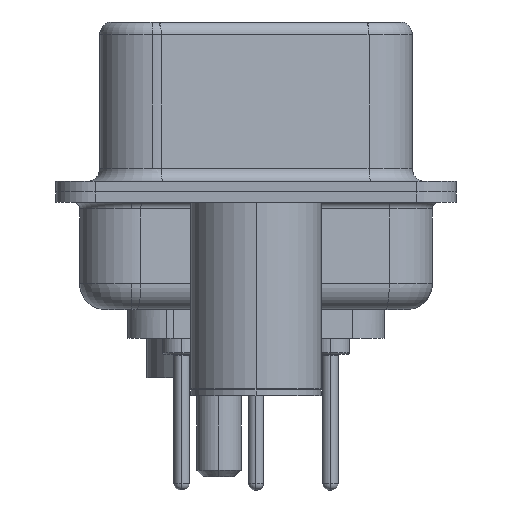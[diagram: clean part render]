
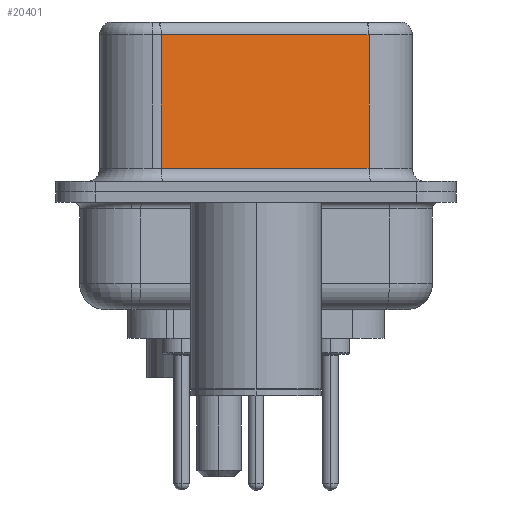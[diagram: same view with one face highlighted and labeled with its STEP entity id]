
A CAD part, left-side view. The second image highlights one B-rep face of the part: STEP entity #20401.
In plain terms, the highlighted planar face has unit normal (-0.985, -0.174, 0).
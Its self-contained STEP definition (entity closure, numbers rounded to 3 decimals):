
#1045 = AXIS2_PLACEMENT_3D ( 'NONE', #29341, #17605, #1717 ) ;
#1717 = DIRECTION ( 'NONE',  ( -0.174, 0.985, 0. ) ) ;
#2095 = CARTESIAN_POINT ( 'NONE',  ( 5.132, -4.322, 0.9 ) ) ;
#3301 = LINE ( 'NONE', #2095, #13790 ) ;
#3924 = CARTESIAN_POINT ( 'NONE',  ( 5.132, -4.322, 0.9 ) ) ;
#5317 = VERTEX_POINT ( 'NONE', #3924 ) ;
#5989 = EDGE_CURVE ( 'NONE', #20471, #5317, #24504, .T. ) ;
#6259 = PLANE ( 'NONE',  #1045 ) ;
#8406 = EDGE_CURVE ( 'NONE', #20471, #17214, #12701, .T. ) ;
#8495 = VECTOR ( 'NONE', #23700, 1000. ) ;
#9767 = DIRECTION ( 'NONE',  ( -0.174, 0.985, 0. ) ) ;
#10896 = CARTESIAN_POINT ( 'NONE',  ( 3.73, 3.628, 0.9 ) ) ;
#10901 = DIRECTION ( 'NONE',  ( 0.174, -0.985, 0. ) ) ;
#11089 = VECTOR ( 'NONE', #12993, 1000. ) ;
#11723 = CARTESIAN_POINT ( 'NONE',  ( 5.132, -4.322, 6.52 ) ) ;
#12054 = EDGE_CURVE ( 'NONE', #17214, #20458, #22404, .T. ) ;
#12107 = CARTESIAN_POINT ( 'NONE',  ( 5.132, -4.322, 6.02 ) ) ;
#12701 = LINE ( 'NONE', #12107, #25792 ) ;
#12714 = ORIENTED_EDGE ( 'NONE', *, *, #22358, .T. ) ;
#12993 = DIRECTION ( 'NONE',  ( 0., 0., -1. ) ) ;
#13790 = VECTOR ( 'NONE', #10901, 1000. ) ;
#15460 = CARTESIAN_POINT ( 'NONE',  ( 5.132, -4.322, 6.02 ) ) ;
#15573 = ORIENTED_EDGE ( 'NONE', *, *, #12054, .T. ) ;
#17214 = VERTEX_POINT ( 'NONE', #24211 ) ;
#17605 = DIRECTION ( 'NONE',  ( 0.985, 0.174, 0. ) ) ;
#18900 = FACE_OUTER_BOUND ( 'NONE', #26830, .T. ) ;
#20401 = ADVANCED_FACE ( 'NONE', ( #18900 ), #6259, .F. ) ;
#20458 = VERTEX_POINT ( 'NONE', #10896 ) ;
#20471 = VERTEX_POINT ( 'NONE', #15460 ) ;
#22358 = EDGE_CURVE ( 'NONE', #20458, #5317, #3301, .T. ) ;
#22404 = LINE ( 'NONE', #24695, #11089 ) ;
#22924 = ORIENTED_EDGE ( 'NONE', *, *, #8406, .T. ) ;
#23700 = DIRECTION ( 'NONE',  ( 0., 0., -1. ) ) ;
#24211 = CARTESIAN_POINT ( 'NONE',  ( 3.73, 3.628, 6.02 ) ) ;
#24504 = LINE ( 'NONE', #11723, #8495 ) ;
#24695 = CARTESIAN_POINT ( 'NONE',  ( 3.73, 3.628, 6.52 ) ) ;
#25792 = VECTOR ( 'NONE', #9767, 1000. ) ;
#26830 = EDGE_LOOP ( 'NONE', ( #29861, #22924, #15573, #12714 ) ) ;
#29341 = CARTESIAN_POINT ( 'NONE',  ( 5.132, -4.322, 6.52 ) ) ;
#29861 = ORIENTED_EDGE ( 'NONE', *, *, #5989, .F. ) ;
